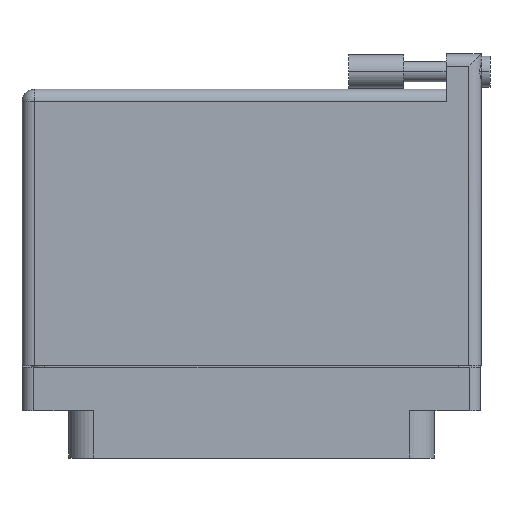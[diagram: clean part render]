
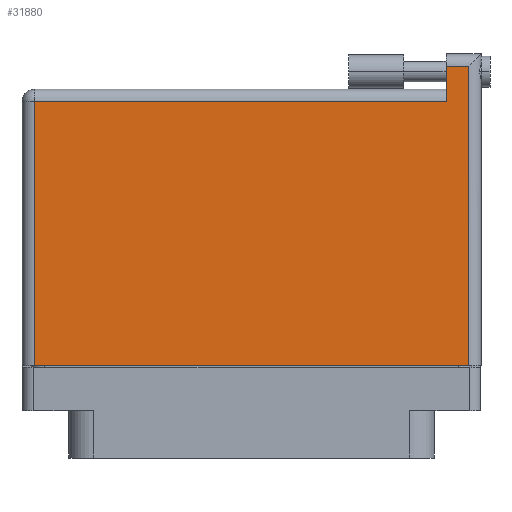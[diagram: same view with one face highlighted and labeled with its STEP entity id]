
A CAD part, front view. The second image highlights one B-rep face of the part: STEP entity #31880.
In plain terms, the highlighted face is planar.
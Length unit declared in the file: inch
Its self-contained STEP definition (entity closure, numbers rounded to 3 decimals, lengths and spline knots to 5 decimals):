
#1200 = VERTEX_POINT ( 'NONE', #38188 ) ;
#1654 = CARTESIAN_POINT ( 'NONE',  ( -1.3, 1.396, 0.4495 ) ) ;
#1773 = VECTOR ( 'NONE', #34227, 39.37008 ) ;
#3226 = ORIENTED_EDGE ( 'NONE', *, *, #10839, .T. ) ;
#3916 = CARTESIAN_POINT ( 'NONE',  ( 1.23, 1.596, 0.4495 ) ) ;
#4199 = CARTESIAN_POINT ( 'NONE',  ( -1.3, 1.466, 0.4495 ) ) ;
#5062 = LINE ( 'NONE', #44609, #44408 ) ;
#5477 = PLANE ( 'NONE',  #6586 ) ;
#5518 = CARTESIAN_POINT ( 'NONE',  ( -1.3, -0.1, 0.4495 ) ) ;
#6144 = DIRECTION ( 'NONE',  ( 1., 0., 0. ) ) ;
#6287 = CARTESIAN_POINT ( 'NONE',  ( 1.103, 1.596, 0.4495 ) ) ;
#6586 = AXIS2_PLACEMENT_3D ( 'NONE', #4199, #8156, #11792 ) ;
#7030 = VERTEX_POINT ( 'NONE', #6287 ) ;
#8156 = DIRECTION ( 'NONE',  ( 0., 0., -1. ) ) ;
#8454 = VECTOR ( 'NONE', #44339, 39.37008 ) ;
#8658 = VECTOR ( 'NONE', #41872, 39.37008 ) ;
#10839 = EDGE_CURVE ( 'NONE', #39747, #17871, #29705, .T. ) ;
#11350 = FACE_OUTER_BOUND ( 'NONE', #18929, .T. ) ;
#11792 = DIRECTION ( 'NONE',  ( -1., 0., 0. ) ) ;
#12952 = CARTESIAN_POINT ( 'NONE',  ( 1.23, -0.1, 0.4495 ) ) ;
#13238 = ORIENTED_EDGE ( 'NONE', *, *, #21976, .T. ) ;
#13439 = CARTESIAN_POINT ( 'NONE',  ( -1.23, -0.1, 0.4495 ) ) ;
#14198 = LINE ( 'NONE', #1654, #1773 ) ;
#15301 = DIRECTION ( 'NONE',  ( -1., 0., 0. ) ) ;
#15392 = ORIENTED_EDGE ( 'NONE', *, *, #15614, .T. ) ;
#15614 = EDGE_CURVE ( 'NONE', #16766, #39747, #15839, .T. ) ;
#15839 = LINE ( 'NONE', #5518, #23853 ) ;
#16766 = VERTEX_POINT ( 'NONE', #13439 ) ;
#17871 = VERTEX_POINT ( 'NONE', #3916 ) ;
#18929 = EDGE_LOOP ( 'NONE', ( #15392, #3226, #25296, #34495, #20320, #13238 ) ) ;
#20320 = ORIENTED_EDGE ( 'NONE', *, *, #27325, .T. ) ;
#21564 = EDGE_CURVE ( 'NONE', #7030, #1200, #40476, .T. ) ;
#21976 = EDGE_CURVE ( 'NONE', #27107, #16766, #5062, .T. ) ;
#23853 = VECTOR ( 'NONE', #6144, 39.37008 ) ;
#25296 = ORIENTED_EDGE ( 'NONE', *, *, #40978, .T. ) ;
#25974 = CARTESIAN_POINT ( 'NONE',  ( -1.3, 1.596, 0.4495 ) ) ;
#27107 = VERTEX_POINT ( 'NONE', #36655 ) ;
#27325 = EDGE_CURVE ( 'NONE', #1200, #27107, #14198, .T. ) ;
#29705 = LINE ( 'NONE', #41567, #8658 ) ;
#31880 = ADVANCED_FACE ( 'NONE', ( #11350 ), #5477, .F. ) ;
#32425 = VECTOR ( 'NONE', #15301, 39.37008 ) ;
#34227 = DIRECTION ( 'NONE',  ( -1., 0., 0. ) ) ;
#34495 = ORIENTED_EDGE ( 'NONE', *, *, #21564, .T. ) ;
#36617 = DIRECTION ( 'NONE',  ( 0., -1., 0. ) ) ;
#36655 = CARTESIAN_POINT ( 'NONE',  ( -1.23, 1.396, 0.4495 ) ) ;
#36958 = CARTESIAN_POINT ( 'NONE',  ( 1.103, 1.666, 0.4495 ) ) ;
#38188 = CARTESIAN_POINT ( 'NONE',  ( 1.103, 1.396, 0.4495 ) ) ;
#38191 = LINE ( 'NONE', #25974, #32425 ) ;
#39747 = VERTEX_POINT ( 'NONE', #12952 ) ;
#40476 = LINE ( 'NONE', #36958, #8454 ) ;
#40978 = EDGE_CURVE ( 'NONE', #17871, #7030, #38191, .T. ) ;
#41567 = CARTESIAN_POINT ( 'NONE',  ( 1.23, 1.666, 0.4495 ) ) ;
#41872 = DIRECTION ( 'NONE',  ( 0., 1., 0. ) ) ;
#44339 = DIRECTION ( 'NONE',  ( 0., -1., 0. ) ) ;
#44408 = VECTOR ( 'NONE', #36617, 39.37008 ) ;
#44609 = CARTESIAN_POINT ( 'NONE',  ( -1.23, -0.1, 0.4495 ) ) ;
